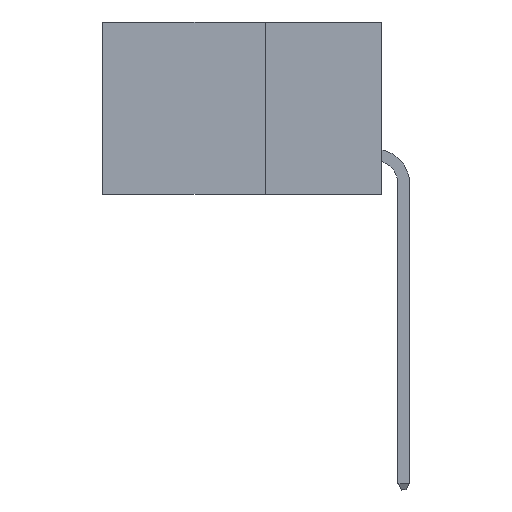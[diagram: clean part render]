
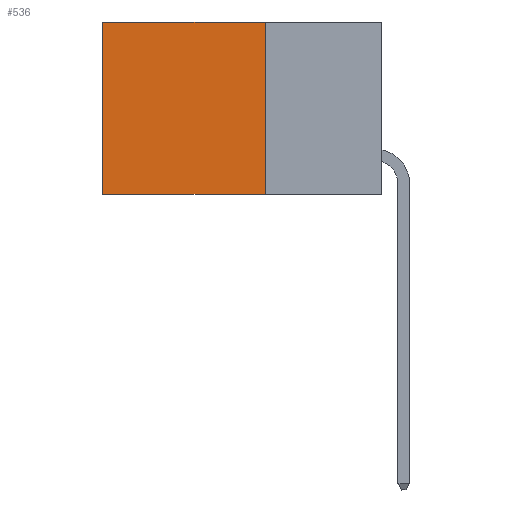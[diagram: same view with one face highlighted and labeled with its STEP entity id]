
A CAD part, left-side view. The second image highlights one B-rep face of the part: STEP entity #536.
In plain terms, the highlighted planar face has unit normal (-1, 0, 0).
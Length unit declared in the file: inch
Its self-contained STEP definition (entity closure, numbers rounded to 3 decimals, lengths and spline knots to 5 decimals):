
#202 = CARTESIAN_POINT ( 'NONE',  ( 0.2875, 0.6, -0.37 ) ) ;
#439 = VECTOR ( 'NONE', #6511, 39.37008 ) ;
#536 = ADVANCED_FACE ( 'NONE', ( #7184 ), #11169, .F. ) ;
#613 = CARTESIAN_POINT ( 'NONE',  ( 0.2875, 0.25, 0. ) ) ;
#1824 = CARTESIAN_POINT ( 'NONE',  ( 0.2875, 0.25, -0.37 ) ) ;
#3470 = DIRECTION ( 'NONE',  ( 0., 0., -1. ) ) ;
#3635 = CARTESIAN_POINT ( 'NONE',  ( 0.2875, 0.25, 0. ) ) ;
#3991 = ORIENTED_EDGE ( 'NONE', *, *, #7306, .F. ) ;
#4223 = ORIENTED_EDGE ( 'NONE', *, *, #16740, .T. ) ;
#4325 = ORIENTED_EDGE ( 'NONE', *, *, #22446, .F. ) ;
#4840 = DIRECTION ( 'NONE',  ( 0., 1., 0. ) ) ;
#5227 = CARTESIAN_POINT ( 'NONE',  ( 0.2875, 0.25, 0. ) ) ;
#5585 = LINE ( 'NONE', #17933, #439 ) ;
#5857 = LINE ( 'NONE', #3635, #13679 ) ;
#6511 = DIRECTION ( 'NONE',  ( 0., 0., -1. ) ) ;
#6629 = LINE ( 'NONE', #613, #10852 ) ;
#7184 = FACE_OUTER_BOUND ( 'NONE', #13065, .T. ) ;
#7261 = LINE ( 'NONE', #12621, #22807 ) ;
#7306 = EDGE_CURVE ( 'NONE', #14956, #21016, #7261, .T. ) ;
#7497 = DIRECTION ( 'NONE',  ( 0., 1., 0. ) ) ;
#7583 = VERTEX_POINT ( 'NONE', #19081 ) ;
#9605 = VERTEX_POINT ( 'NONE', #18052 ) ;
#10076 = EDGE_CURVE ( 'NONE', #7583, #21016, #5585, .T. ) ;
#10852 = VECTOR ( 'NONE', #21530, 39.37008 ) ;
#11169 = PLANE ( 'NONE',  #20366 ) ;
#12621 = CARTESIAN_POINT ( 'NONE',  ( 0.2875, 0.25, -0.37 ) ) ;
#13065 = EDGE_LOOP ( 'NONE', ( #21594, #3991, #4325, #4223 ) ) ;
#13679 = VECTOR ( 'NONE', #7497, 39.37008 ) ;
#14956 = VERTEX_POINT ( 'NONE', #1824 ) ;
#14965 = DIRECTION ( 'NONE',  ( 1., 0., 0. ) ) ;
#16740 = EDGE_CURVE ( 'NONE', #9605, #7583, #5857, .T. ) ;
#17933 = CARTESIAN_POINT ( 'NONE',  ( 0.2875, 0.6, 0. ) ) ;
#18052 = CARTESIAN_POINT ( 'NONE',  ( 0.2875, 0.25, 0. ) ) ;
#19081 = CARTESIAN_POINT ( 'NONE',  ( 0.2875, 0.6, 0. ) ) ;
#20366 = AXIS2_PLACEMENT_3D ( 'NONE', #5227, #14965, #3470 ) ;
#21016 = VERTEX_POINT ( 'NONE', #202 ) ;
#21530 = DIRECTION ( 'NONE',  ( 0., 0., -1. ) ) ;
#21594 = ORIENTED_EDGE ( 'NONE', *, *, #10076, .T. ) ;
#22446 = EDGE_CURVE ( 'NONE', #9605, #14956, #6629, .T. ) ;
#22807 = VECTOR ( 'NONE', #4840, 39.37008 ) ;
